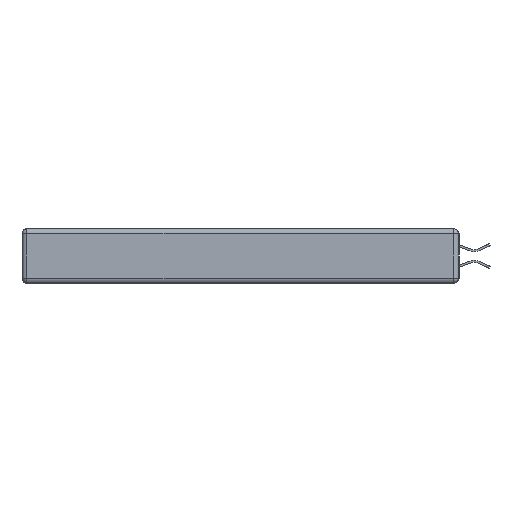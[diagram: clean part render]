
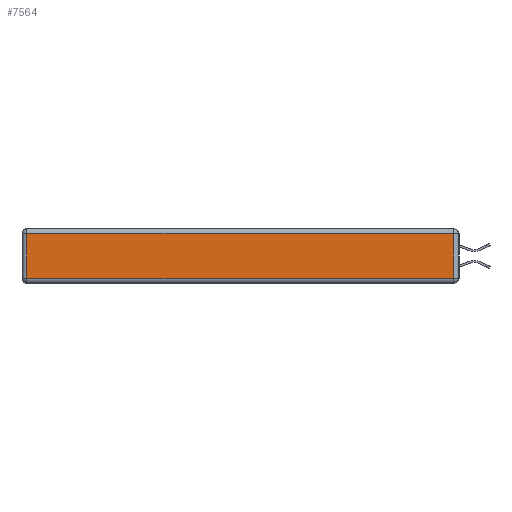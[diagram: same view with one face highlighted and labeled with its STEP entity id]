
A CAD part, left-side view. The second image highlights one B-rep face of the part: STEP entity #7564.
In plain terms, the highlighted planar face has unit normal (-1, 0, 0).
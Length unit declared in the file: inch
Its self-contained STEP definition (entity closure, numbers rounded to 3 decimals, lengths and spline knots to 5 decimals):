
#580 = EDGE_CURVE ( 'NONE', #28883, #30048, #8347, .T. ) ;
#648 = EDGE_LOOP ( 'NONE', ( #27501, #769, #24240, #30902 ) ) ;
#769 = ORIENTED_EDGE ( 'NONE', *, *, #14651, .T. ) ;
#2443 = DIRECTION ( 'NONE',  ( -1., 0., 0. ) ) ;
#2717 = EDGE_CURVE ( 'NONE', #30048, #29888, #27630, .T. ) ;
#4956 = CARTESIAN_POINT ( 'NONE',  ( 0., 0., -0.343 ) ) ;
#7390 = DIRECTION ( 'NONE',  ( 0., 0., 1. ) ) ;
#7564 = ADVANCED_FACE ( 'NONE', ( #9416 ), #16971, .T. ) ;
#7938 = CARTESIAN_POINT ( 'NONE',  ( 0., 0.03, -0.03 ) ) ;
#8347 = LINE ( 'NONE', #12010, #27164 ) ;
#9019 = VERTEX_POINT ( 'NONE', #7938 ) ;
#9416 = FACE_OUTER_BOUND ( 'NONE', #648, .T. ) ;
#11455 = CARTESIAN_POINT ( 'NONE',  ( 0., 2.72, -0.313 ) ) ;
#12010 = CARTESIAN_POINT ( 'NONE',  ( 0., 2.72, -0.343 ) ) ;
#13745 = DIRECTION ( 'NONE',  ( 0., 0., 1. ) ) ;
#14072 = VECTOR ( 'NONE', #15258, 39.37008 ) ;
#14651 = EDGE_CURVE ( 'NONE', #29888, #9019, #23407, .T. ) ;
#15258 = DIRECTION ( 'NONE',  ( 0., 1., 0. ) ) ;
#15361 = CARTESIAN_POINT ( 'NONE',  ( 0., 2.75, -0.03 ) ) ;
#15944 = CARTESIAN_POINT ( 'NONE',  ( 0., 0.03, -0.343 ) ) ;
#16971 = PLANE ( 'NONE',  #21477 ) ;
#17001 = VECTOR ( 'NONE', #13745, 39.37008 ) ;
#19936 = EDGE_CURVE ( 'NONE', #9019, #28883, #27577, .T. ) ;
#21477 = AXIS2_PLACEMENT_3D ( 'NONE', #4956, #2443, #7390 ) ;
#21751 = CARTESIAN_POINT ( 'NONE',  ( 0., 0., -0.313 ) ) ;
#22787 = VECTOR ( 'NONE', #26659, 39.37008 ) ;
#22931 = CARTESIAN_POINT ( 'NONE',  ( 0., 0.03, -0.313 ) ) ;
#23407 = LINE ( 'NONE', #15944, #17001 ) ;
#24240 = ORIENTED_EDGE ( 'NONE', *, *, #19936, .T. ) ;
#26659 = DIRECTION ( 'NONE',  ( 0., -1., 0. ) ) ;
#27164 = VECTOR ( 'NONE', #29427, 39.37008 ) ;
#27501 = ORIENTED_EDGE ( 'NONE', *, *, #2717, .T. ) ;
#27577 = LINE ( 'NONE', #15361, #14072 ) ;
#27630 = LINE ( 'NONE', #21751, #22787 ) ;
#28883 = VERTEX_POINT ( 'NONE', #31155 ) ;
#29427 = DIRECTION ( 'NONE',  ( 0., 0., -1. ) ) ;
#29888 = VERTEX_POINT ( 'NONE', #22931 ) ;
#30048 = VERTEX_POINT ( 'NONE', #11455 ) ;
#30902 = ORIENTED_EDGE ( 'NONE', *, *, #580, .T. ) ;
#31155 = CARTESIAN_POINT ( 'NONE',  ( 0., 2.72, -0.03 ) ) ;
